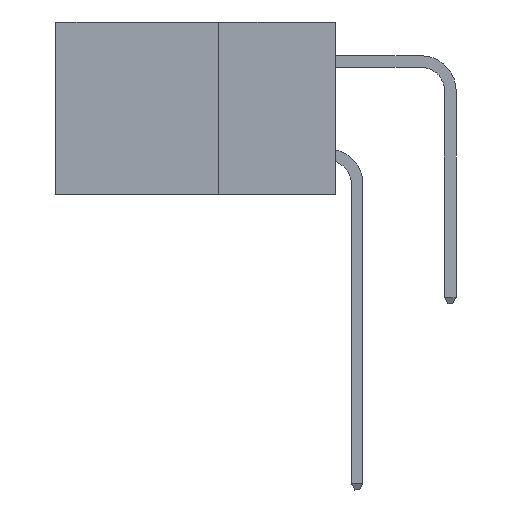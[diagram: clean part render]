
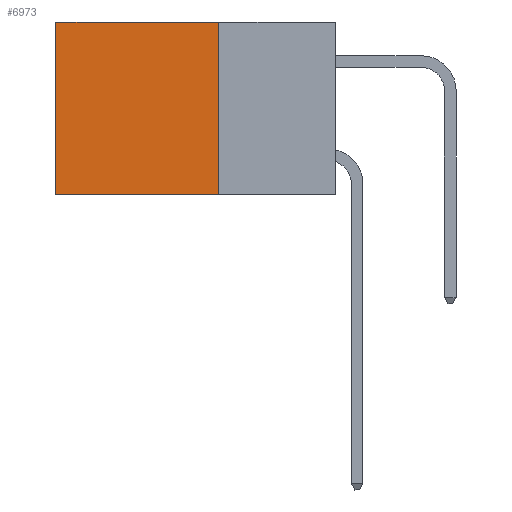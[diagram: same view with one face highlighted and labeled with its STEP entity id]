
A CAD part, left-side view. The second image highlights one B-rep face of the part: STEP entity #6973.
In plain terms, the highlighted planar face has unit normal (-1, 0, 0).
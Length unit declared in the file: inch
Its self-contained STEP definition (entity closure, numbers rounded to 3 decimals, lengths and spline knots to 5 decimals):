
#1557 = LINE ( 'NONE', #3842, #21845 ) ;
#1733 = AXIS2_PLACEMENT_3D ( 'NONE', #8146, #28756, #17564 ) ;
#3657 = VECTOR ( 'NONE', #21717, 39.37008 ) ;
#3842 = CARTESIAN_POINT ( 'NONE',  ( 0.2875, 0.25, 0. ) ) ;
#3985 = VERTEX_POINT ( 'NONE', #26280 ) ;
#3998 = ORIENTED_EDGE ( 'NONE', *, *, #14752, .T. ) ;
#4324 = VERTEX_POINT ( 'NONE', #15993 ) ;
#5466 = CARTESIAN_POINT ( 'NONE',  ( 0.2875, 0.25, -0.37 ) ) ;
#5671 = EDGE_CURVE ( 'NONE', #15286, #4324, #11058, .T. ) ;
#6973 = ADVANCED_FACE ( 'NONE', ( #10972 ), #24247, .F. ) ;
#8146 = CARTESIAN_POINT ( 'NONE',  ( 0.2875, 0.25, 0. ) ) ;
#8917 = EDGE_LOOP ( 'NONE', ( #25022, #20784, #20277, #3998 ) ) ;
#9402 = LINE ( 'NONE', #14714, #3657 ) ;
#10757 = EDGE_CURVE ( 'NONE', #3985, #4324, #9402, .T. ) ;
#10768 = DIRECTION ( 'NONE',  ( 0., 0., -1. ) ) ;
#10972 = FACE_OUTER_BOUND ( 'NONE', #8917, .T. ) ;
#11058 = LINE ( 'NONE', #5466, #18305 ) ;
#12224 = EDGE_CURVE ( 'NONE', #16183, #15286, #21675, .T. ) ;
#14714 = CARTESIAN_POINT ( 'NONE',  ( 0.2875, 0.6, 0. ) ) ;
#14752 = EDGE_CURVE ( 'NONE', #16183, #3985, #1557, .T. ) ;
#15286 = VERTEX_POINT ( 'NONE', #21587 ) ;
#15993 = CARTESIAN_POINT ( 'NONE',  ( 0.2875, 0.6, -0.37 ) ) ;
#16183 = VERTEX_POINT ( 'NONE', #26087 ) ;
#16959 = VECTOR ( 'NONE', #10768, 39.37008 ) ;
#17564 = DIRECTION ( 'NONE',  ( 0., 0., -1. ) ) ;
#18305 = VECTOR ( 'NONE', #24198, 39.37008 ) ;
#20055 = DIRECTION ( 'NONE',  ( 0., 1., 0. ) ) ;
#20277 = ORIENTED_EDGE ( 'NONE', *, *, #12224, .F. ) ;
#20784 = ORIENTED_EDGE ( 'NONE', *, *, #5671, .F. ) ;
#21587 = CARTESIAN_POINT ( 'NONE',  ( 0.2875, 0.25, -0.37 ) ) ;
#21675 = LINE ( 'NONE', #26998, #16959 ) ;
#21717 = DIRECTION ( 'NONE',  ( 0., 0., -1. ) ) ;
#21845 = VECTOR ( 'NONE', #20055, 39.37008 ) ;
#24198 = DIRECTION ( 'NONE',  ( 0., 1., 0. ) ) ;
#24247 = PLANE ( 'NONE',  #1733 ) ;
#25022 = ORIENTED_EDGE ( 'NONE', *, *, #10757, .T. ) ;
#26087 = CARTESIAN_POINT ( 'NONE',  ( 0.2875, 0.25, 0. ) ) ;
#26280 = CARTESIAN_POINT ( 'NONE',  ( 0.2875, 0.6, 0. ) ) ;
#26998 = CARTESIAN_POINT ( 'NONE',  ( 0.2875, 0.25, 0. ) ) ;
#28756 = DIRECTION ( 'NONE',  ( 1., 0., 0. ) ) ;
